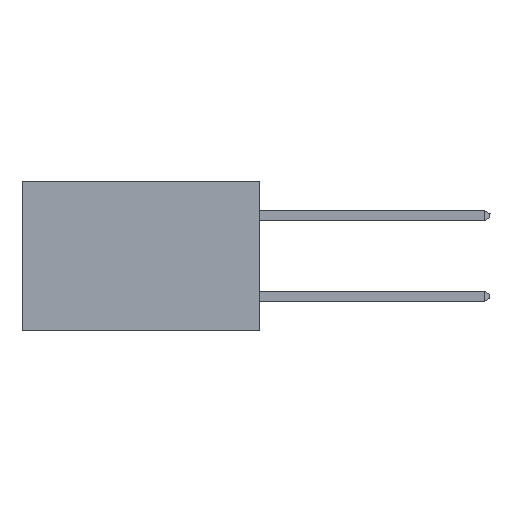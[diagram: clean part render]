
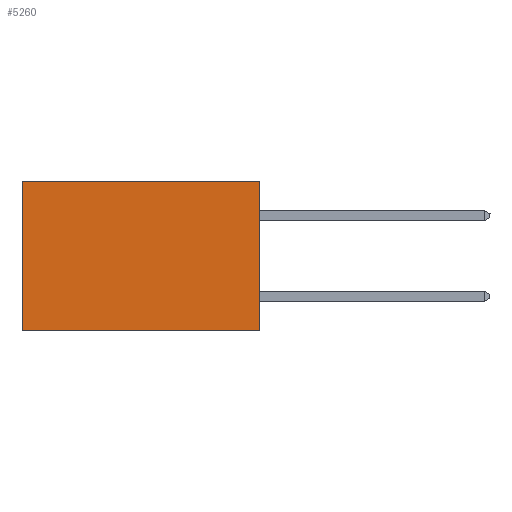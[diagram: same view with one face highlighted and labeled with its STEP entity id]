
A CAD part, left-side view. The second image highlights one B-rep face of the part: STEP entity #5260.
In plain terms, the highlighted planar face has unit normal (-1, 0, 0).
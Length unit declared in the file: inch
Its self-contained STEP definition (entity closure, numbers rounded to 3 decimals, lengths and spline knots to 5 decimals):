
#128 = CARTESIAN_POINT ( 'NONE',  ( 0.277, 0.59, -0.37 ) ) ;
#525 = LINE ( 'NONE', #2481, #6665 ) ;
#577 = CARTESIAN_POINT ( 'NONE',  ( 0.277, 0.59, -0.37 ) ) ;
#943 = VERTEX_POINT ( 'NONE', #577 ) ;
#1290 = EDGE_LOOP ( 'NONE', ( #5690, #7431, #4109, #4196 ) ) ;
#1903 = VERTEX_POINT ( 'NONE', #2497 ) ;
#2481 = CARTESIAN_POINT ( 'NONE',  ( 0.277, 0., -0.37 ) ) ;
#2497 = CARTESIAN_POINT ( 'NONE',  ( 0.277, 0., -0.37 ) ) ;
#2618 = EDGE_CURVE ( 'NONE', #8003, #3264, #4019, .T. ) ;
#3095 = VECTOR ( 'NONE', #8953, 39.37008 ) ;
#3239 = DIRECTION ( 'NONE',  ( 0., 0., -1. ) ) ;
#3264 = VERTEX_POINT ( 'NONE', #7575 ) ;
#3708 = DIRECTION ( 'NONE',  ( 0., 1., 0. ) ) ;
#3756 = CARTESIAN_POINT ( 'NONE',  ( 0.277, 0., -0.37 ) ) ;
#4019 = LINE ( 'NONE', #8443, #3095 ) ;
#4109 = ORIENTED_EDGE ( 'NONE', *, *, #4745, .F. ) ;
#4196 = ORIENTED_EDGE ( 'NONE', *, *, #2618, .T. ) ;
#4403 = AXIS2_PLACEMENT_3D ( 'NONE', #3756, #8438, #4508 ) ;
#4462 = CARTESIAN_POINT ( 'NONE',  ( 0.277, 0., -0.37 ) ) ;
#4508 = DIRECTION ( 'NONE',  ( 0., 0., -1. ) ) ;
#4540 = VECTOR ( 'NONE', #3708, 39.37008 ) ;
#4745 = EDGE_CURVE ( 'NONE', #8003, #1903, #525, .T. ) ;
#5193 = LINE ( 'NONE', #128, #6731 ) ;
#5260 = ADVANCED_FACE ( 'NONE', ( #5837 ), #7169, .F. ) ;
#5489 = DIRECTION ( 'NONE',  ( 0., 0., -1. ) ) ;
#5690 = ORIENTED_EDGE ( 'NONE', *, *, #6597, .T. ) ;
#5837 = FACE_OUTER_BOUND ( 'NONE', #1290, .T. ) ;
#6086 = CARTESIAN_POINT ( 'NONE',  ( 0.277, 0., 0. ) ) ;
#6102 = EDGE_CURVE ( 'NONE', #1903, #943, #8074, .T. ) ;
#6597 = EDGE_CURVE ( 'NONE', #3264, #943, #5193, .T. ) ;
#6665 = VECTOR ( 'NONE', #3239, 39.37008 ) ;
#6731 = VECTOR ( 'NONE', #5489, 39.37008 ) ;
#7169 = PLANE ( 'NONE',  #4403 ) ;
#7431 = ORIENTED_EDGE ( 'NONE', *, *, #6102, .F. ) ;
#7575 = CARTESIAN_POINT ( 'NONE',  ( 0.277, 0.59, 0. ) ) ;
#8003 = VERTEX_POINT ( 'NONE', #6086 ) ;
#8074 = LINE ( 'NONE', #4462, #4540 ) ;
#8438 = DIRECTION ( 'NONE',  ( 1., 0., 0. ) ) ;
#8443 = CARTESIAN_POINT ( 'NONE',  ( 0.277, 0., 0. ) ) ;
#8953 = DIRECTION ( 'NONE',  ( 0., 1., 0. ) ) ;
